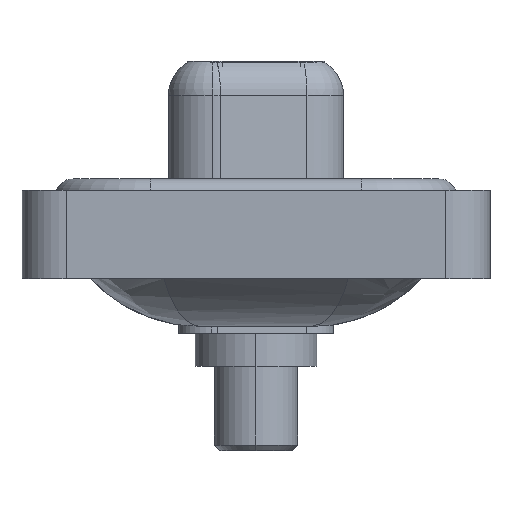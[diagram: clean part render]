
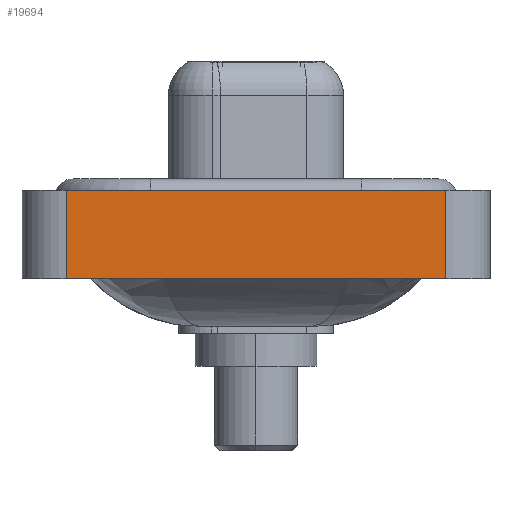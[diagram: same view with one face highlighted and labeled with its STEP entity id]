
A CAD part, left-side view. The second image highlights one B-rep face of the part: STEP entity #19694.
In plain terms, the highlighted planar face has unit normal (-1, 0, 0).
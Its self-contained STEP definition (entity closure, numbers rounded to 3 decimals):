
#1542 = LINE ( 'NONE', #12610, #5392 ) ;
#2096 = VERTEX_POINT ( 'NONE', #5993 ) ;
#3407 = CARTESIAN_POINT ( 'NONE',  ( -7.35, 8.55, 0.4 ) ) ;
#4714 = ORIENTED_EDGE ( 'NONE', *, *, #18169, .F. ) ;
#5120 = VECTOR ( 'NONE', #9699, 1000. ) ;
#5392 = VECTOR ( 'NONE', #14098, 1000. ) ;
#5707 = AXIS2_PLACEMENT_3D ( 'NONE', #19391, #16240, #7520 ) ;
#5940 = ORIENTED_EDGE ( 'NONE', *, *, #14995, .T. ) ;
#5993 = CARTESIAN_POINT ( 'NONE',  ( -7.35, -8.55, 0.4 ) ) ;
#6022 = CARTESIAN_POINT ( 'NONE',  ( -7.35, -8.55, -3.6 ) ) ;
#6339 = CARTESIAN_POINT ( 'NONE',  ( -7.35, 8.55, -3.6 ) ) ;
#6468 = LINE ( 'NONE', #11475, #7808 ) ;
#6594 = FACE_OUTER_BOUND ( 'NONE', #16158, .T. ) ;
#7520 = DIRECTION ( 'NONE',  ( 0., 0., 1. ) ) ;
#7808 = VECTOR ( 'NONE', #17785, 1000. ) ;
#8146 = LINE ( 'NONE', #20531, #5120 ) ;
#8263 = CARTESIAN_POINT ( 'NONE',  ( -7.35, -8.55, -3.6 ) ) ;
#8385 = ORIENTED_EDGE ( 'NONE', *, *, #17288, .T. ) ;
#9244 = DIRECTION ( 'NONE',  ( 0., 0., 1. ) ) ;
#9464 = VECTOR ( 'NONE', #9244, 1000. ) ;
#9559 = VERTEX_POINT ( 'NONE', #3407 ) ;
#9699 = DIRECTION ( 'NONE',  ( 0., -1., 0. ) ) ;
#11475 = CARTESIAN_POINT ( 'NONE',  ( -7.35, -8.55, 0.4 ) ) ;
#12292 = LINE ( 'NONE', #6022, #9464 ) ;
#12610 = CARTESIAN_POINT ( 'NONE',  ( -7.35, 8.55, -3.6 ) ) ;
#12980 = PLANE ( 'NONE',  #5707 ) ;
#13336 = EDGE_CURVE ( 'NONE', #15451, #9559, #1542, .T. ) ;
#14098 = DIRECTION ( 'NONE',  ( 0., 0., 1. ) ) ;
#14995 = EDGE_CURVE ( 'NONE', #15451, #19659, #8146, .T. ) ;
#15451 = VERTEX_POINT ( 'NONE', #6339 ) ;
#16158 = EDGE_LOOP ( 'NONE', ( #8385, #4714, #19070, #5940 ) ) ;
#16240 = DIRECTION ( 'NONE',  ( -1., 0., 0. ) ) ;
#17288 = EDGE_CURVE ( 'NONE', #19659, #2096, #12292, .T. ) ;
#17785 = DIRECTION ( 'NONE',  ( 0., -1., 0. ) ) ;
#18169 = EDGE_CURVE ( 'NONE', #9559, #2096, #6468, .T. ) ;
#19070 = ORIENTED_EDGE ( 'NONE', *, *, #13336, .F. ) ;
#19391 = CARTESIAN_POINT ( 'NONE',  ( -7.35, -8.55, -3.6 ) ) ;
#19659 = VERTEX_POINT ( 'NONE', #8263 ) ;
#19694 = ADVANCED_FACE ( 'NONE', ( #6594 ), #12980, .T. ) ;
#20531 = CARTESIAN_POINT ( 'NONE',  ( -7.35, -8.55, -3.6 ) ) ;
